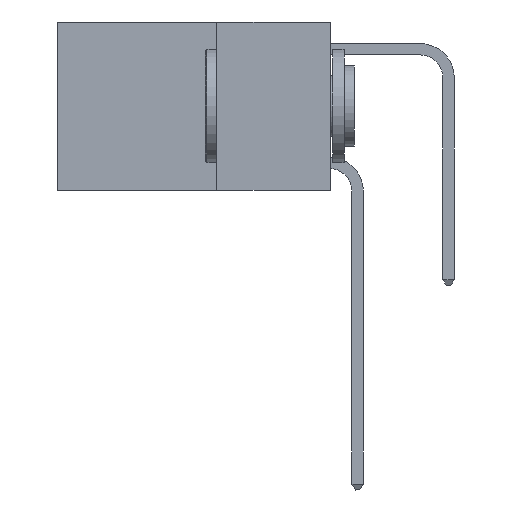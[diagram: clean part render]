
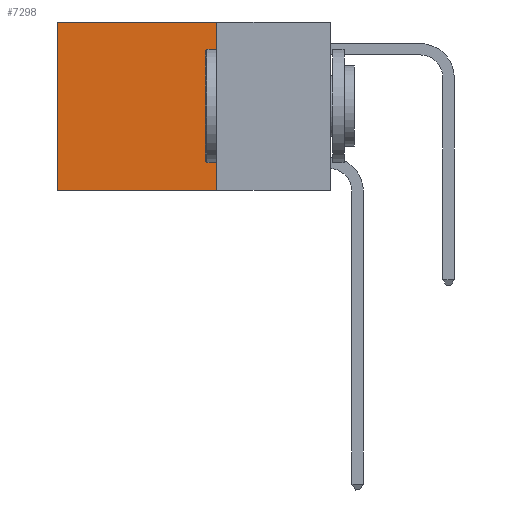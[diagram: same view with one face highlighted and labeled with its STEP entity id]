
A CAD part, left-side view. The second image highlights one B-rep face of the part: STEP entity #7298.
In plain terms, the highlighted planar face has unit normal (-1, 0, 0).
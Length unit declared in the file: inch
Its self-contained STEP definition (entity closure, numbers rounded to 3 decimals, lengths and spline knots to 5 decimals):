
#355 = CARTESIAN_POINT ( 'NONE',  ( 0.2625, 0.6, -0.37 ) ) ;
#660 = ORIENTED_EDGE ( 'NONE', *, *, #10404, .T. ) ;
#701 = LINE ( 'NONE', #2536, #18951 ) ;
#863 = DIRECTION ( 'NONE',  ( 0., 0., -1. ) ) ;
#2536 = CARTESIAN_POINT ( 'NONE',  ( 0.2625, 0.25, 0. ) ) ;
#2558 = EDGE_LOOP ( 'NONE', ( #660, #8611, #10764, #2697 ) ) ;
#2697 = ORIENTED_EDGE ( 'NONE', *, *, #5630, .T. ) ;
#3818 = VERTEX_POINT ( 'NONE', #15861 ) ;
#4853 = EDGE_CURVE ( 'NONE', #3818, #7123, #9458, .T. ) ;
#5630 = EDGE_CURVE ( 'NONE', #3818, #9422, #701, .T. ) ;
#6078 = LINE ( 'NONE', #20770, #16101 ) ;
#6081 = CARTESIAN_POINT ( 'NONE',  ( 0.2625, 0.25, 0. ) ) ;
#6680 = LINE ( 'NONE', #18106, #10399 ) ;
#7123 = VERTEX_POINT ( 'NONE', #10423 ) ;
#7298 = ADVANCED_FACE ( 'NONE', ( #14592 ), #12612, .F. ) ;
#7874 = VERTEX_POINT ( 'NONE', #355 ) ;
#8611 = ORIENTED_EDGE ( 'NONE', *, *, #14284, .F. ) ;
#8969 = DIRECTION ( 'NONE',  ( 0., 1., 0. ) ) ;
#9422 = VERTEX_POINT ( 'NONE', #10592 ) ;
#9458 = LINE ( 'NONE', #9780, #16580 ) ;
#9780 = CARTESIAN_POINT ( 'NONE',  ( 0.2625, 0.25, 0. ) ) ;
#10399 = VECTOR ( 'NONE', #19839, 39.37008 ) ;
#10404 = EDGE_CURVE ( 'NONE', #9422, #7874, #6680, .T. ) ;
#10423 = CARTESIAN_POINT ( 'NONE',  ( 0.2625, 0.25, -0.37 ) ) ;
#10592 = CARTESIAN_POINT ( 'NONE',  ( 0.2625, 0.6, 0. ) ) ;
#10764 = ORIENTED_EDGE ( 'NONE', *, *, #4853, .F. ) ;
#12612 = PLANE ( 'NONE',  #18348 ) ;
#12747 = DIRECTION ( 'NONE',  ( 0., 0., -1. ) ) ;
#12832 = DIRECTION ( 'NONE',  ( 1., 0., 0. ) ) ;
#14284 = EDGE_CURVE ( 'NONE', #7123, #7874, #6078, .T. ) ;
#14372 = DIRECTION ( 'NONE',  ( 0., 1., 0. ) ) ;
#14592 = FACE_OUTER_BOUND ( 'NONE', #2558, .T. ) ;
#15861 = CARTESIAN_POINT ( 'NONE',  ( 0.2625, 0.25, 0. ) ) ;
#16101 = VECTOR ( 'NONE', #14372, 39.37008 ) ;
#16580 = VECTOR ( 'NONE', #12747, 39.37008 ) ;
#18106 = CARTESIAN_POINT ( 'NONE',  ( 0.2625, 0.6, 0. ) ) ;
#18348 = AXIS2_PLACEMENT_3D ( 'NONE', #6081, #12832, #863 ) ;
#18951 = VECTOR ( 'NONE', #8969, 39.37008 ) ;
#19839 = DIRECTION ( 'NONE',  ( 0., 0., -1. ) ) ;
#20770 = CARTESIAN_POINT ( 'NONE',  ( 0.2625, 0.25, -0.37 ) ) ;
